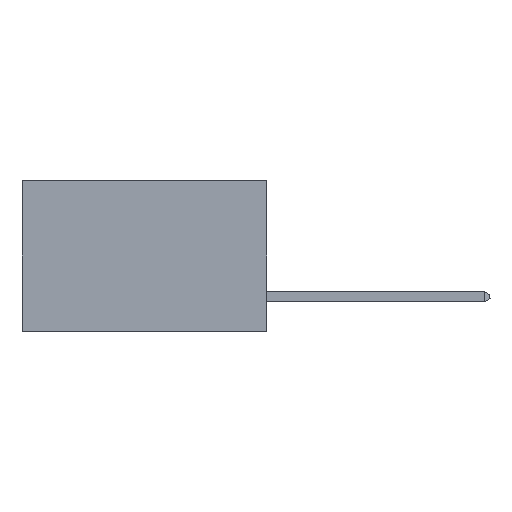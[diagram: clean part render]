
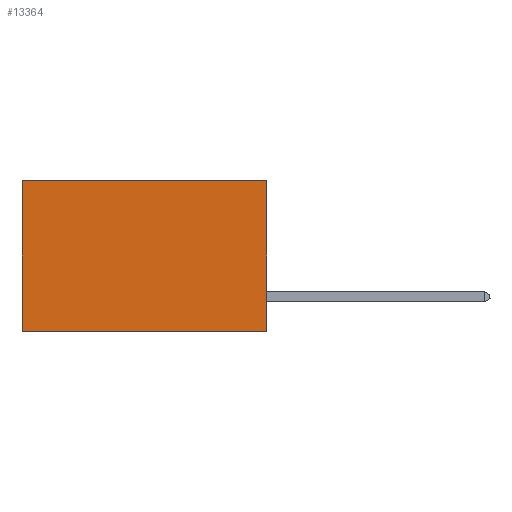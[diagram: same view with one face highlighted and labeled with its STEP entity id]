
A CAD part, left-side view. The second image highlights one B-rep face of the part: STEP entity #13364.
In plain terms, the highlighted planar face has unit normal (-1, 0, 0).
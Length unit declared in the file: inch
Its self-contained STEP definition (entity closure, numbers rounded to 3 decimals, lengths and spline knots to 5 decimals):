
#143 = CARTESIAN_POINT ( 'NONE',  ( 0.2875, 0.6, 0. ) ) ;
#739 = AXIS2_PLACEMENT_3D ( 'NONE', #4049, #1211, #18023 ) ;
#1211 = DIRECTION ( 'NONE',  ( 1., 0., 0. ) ) ;
#2170 = CARTESIAN_POINT ( 'NONE',  ( 0.2875, 0.6, 0. ) ) ;
#2221 = CARTESIAN_POINT ( 'NONE',  ( 0.2875, 0., -0.37 ) ) ;
#2403 = FACE_OUTER_BOUND ( 'NONE', #17451, .T. ) ;
#2407 = VECTOR ( 'NONE', #5922, 39.37008 ) ;
#2590 = EDGE_CURVE ( 'NONE', #5880, #5189, #10903, .T. ) ;
#3656 = VERTEX_POINT ( 'NONE', #2221 ) ;
#3718 = EDGE_CURVE ( 'NONE', #3656, #15741, #3944, .T. ) ;
#3944 = LINE ( 'NONE', #14464, #2407 ) ;
#4049 = CARTESIAN_POINT ( 'NONE',  ( 0.2875, 0., 0. ) ) ;
#4632 = DIRECTION ( 'NONE',  ( 0., 0., -1. ) ) ;
#4636 = VECTOR ( 'NONE', #8493, 39.37008 ) ;
#5189 = VERTEX_POINT ( 'NONE', #2170 ) ;
#5880 = VERTEX_POINT ( 'NONE', #12111 ) ;
#5922 = DIRECTION ( 'NONE',  ( 0., 1., 0. ) ) ;
#6882 = PLANE ( 'NONE',  #739 ) ;
#7131 = VECTOR ( 'NONE', #10096, 39.37008 ) ;
#8130 = ORIENTED_EDGE ( 'NONE', *, *, #2590, .T. ) ;
#8313 = VECTOR ( 'NONE', #4632, 39.37008 ) ;
#8444 = LINE ( 'NONE', #143, #7131 ) ;
#8493 = DIRECTION ( 'NONE',  ( 0., 1., 0. ) ) ;
#10096 = DIRECTION ( 'NONE',  ( 0., 0., -1. ) ) ;
#10106 = ORIENTED_EDGE ( 'NONE', *, *, #3718, .F. ) ;
#10903 = LINE ( 'NONE', #11195, #4636 ) ;
#11195 = CARTESIAN_POINT ( 'NONE',  ( 0.2875, 0., 0. ) ) ;
#11702 = LINE ( 'NONE', #12011, #8313 ) ;
#12011 = CARTESIAN_POINT ( 'NONE',  ( 0.2875, 0., 0. ) ) ;
#12111 = CARTESIAN_POINT ( 'NONE',  ( 0.2875, 0., 0. ) ) ;
#12269 = ORIENTED_EDGE ( 'NONE', *, *, #14405, .F. ) ;
#12272 = EDGE_CURVE ( 'NONE', #5189, #15741, #8444, .T. ) ;
#12418 = ORIENTED_EDGE ( 'NONE', *, *, #12272, .T. ) ;
#13247 = CARTESIAN_POINT ( 'NONE',  ( 0.2875, 0.6, -0.37 ) ) ;
#13364 = ADVANCED_FACE ( 'NONE', ( #2403 ), #6882, .F. ) ;
#14405 = EDGE_CURVE ( 'NONE', #5880, #3656, #11702, .T. ) ;
#14464 = CARTESIAN_POINT ( 'NONE',  ( 0.2875, 0., -0.37 ) ) ;
#15741 = VERTEX_POINT ( 'NONE', #13247 ) ;
#17451 = EDGE_LOOP ( 'NONE', ( #12418, #10106, #12269, #8130 ) ) ;
#18023 = DIRECTION ( 'NONE',  ( 0., 0., -1. ) ) ;
